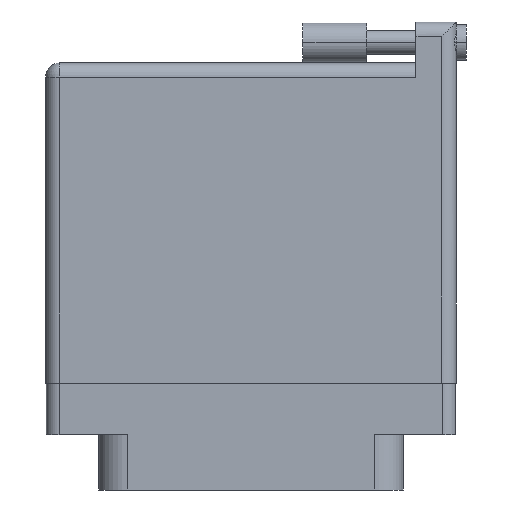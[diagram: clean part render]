
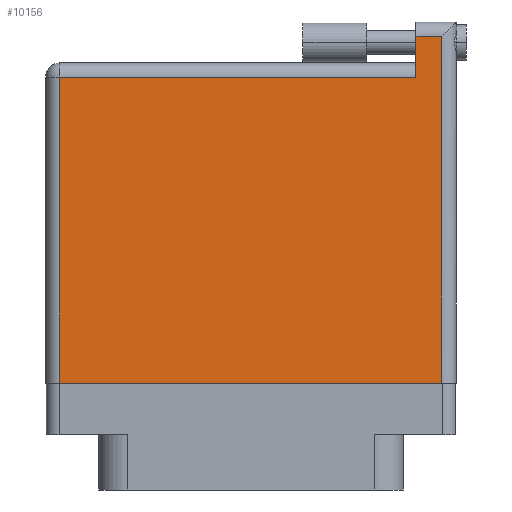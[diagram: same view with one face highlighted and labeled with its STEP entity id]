
A CAD part, front view. The second image highlights one B-rep face of the part: STEP entity #10156.
In plain terms, the highlighted face is planar.
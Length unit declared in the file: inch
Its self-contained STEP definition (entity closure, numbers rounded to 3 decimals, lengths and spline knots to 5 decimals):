
#523 = EDGE_CURVE ( 'NONE', #22296, #26404, #22113, .T. ) ;
#1125 = EDGE_CURVE ( 'NONE', #31940, #37923, #8595, .T. ) ;
#1723 = EDGE_CURVE ( 'NONE', #33157, #22296, #33054, .T. ) ;
#2141 = ORIENTED_EDGE ( 'NONE', *, *, #5294, .T. ) ;
#2783 = CARTESIAN_POINT ( 'NONE',  ( -0.934, -0.1, 0.4495 ) ) ;
#4022 = CARTESIAN_POINT ( 'NONE',  ( -0.934, -0.1, 0.4495 ) ) ;
#4082 = CARTESIAN_POINT ( 'NONE',  ( 0.934, 1.596, 0.4495 ) ) ;
#4830 = EDGE_CURVE ( 'NONE', #34901, #31940, #13661, .T. ) ;
#5192 = DIRECTION ( 'NONE',  ( 0., -1., 0. ) ) ;
#5294 = EDGE_CURVE ( 'NONE', #26404, #34901, #19897, .T. ) ;
#7741 = DIRECTION ( 'NONE',  ( -1., 0., 0. ) ) ;
#7782 = LINE ( 'NONE', #10392, #11637 ) ;
#8595 = LINE ( 'NONE', #8873, #16275 ) ;
#8873 = CARTESIAN_POINT ( 'NONE',  ( -1.004, -0.1, 0.4495 ) ) ;
#8925 = EDGE_CURVE ( 'NONE', #37923, #33157, #7782, .T. ) ;
#10156 = ADVANCED_FACE ( 'NONE', ( #24066 ), #29794, .F. ) ;
#10392 = CARTESIAN_POINT ( 'NONE',  ( 0.934, 1.666, 0.4495 ) ) ;
#11612 = CARTESIAN_POINT ( 'NONE',  ( 0.807, 1.596, 0.4495 ) ) ;
#11637 = VECTOR ( 'NONE', #13107, 39.37008 ) ;
#12786 = ORIENTED_EDGE ( 'NONE', *, *, #523, .T. ) ;
#12849 = VECTOR ( 'NONE', #7741, 39.37008 ) ;
#13107 = DIRECTION ( 'NONE',  ( 0., 1., 0. ) ) ;
#13513 = ORIENTED_EDGE ( 'NONE', *, *, #4830, .T. ) ;
#13623 = VECTOR ( 'NONE', #33402, 39.37008 ) ;
#13661 = LINE ( 'NONE', #2783, #19934 ) ;
#14086 = CARTESIAN_POINT ( 'NONE',  ( 0.807, 1.666, 0.4495 ) ) ;
#14533 = CARTESIAN_POINT ( 'NONE',  ( -1.004, 1.466, 0.4495 ) ) ;
#16275 = VECTOR ( 'NONE', #39687, 39.37008 ) ;
#17135 = CARTESIAN_POINT ( 'NONE',  ( -1.004, 1.596, 0.4495 ) ) ;
#17909 = CARTESIAN_POINT ( 'NONE',  ( 0.807, 1.396, 0.4495 ) ) ;
#17913 = DIRECTION ( 'NONE',  ( 0., 0., -1. ) ) ;
#18087 = CARTESIAN_POINT ( 'NONE',  ( -1.004, 1.396, 0.4495 ) ) ;
#19897 = LINE ( 'NONE', #18087, #13623 ) ;
#19934 = VECTOR ( 'NONE', #36561, 39.37008 ) ;
#20085 = ORIENTED_EDGE ( 'NONE', *, *, #8925, .T. ) ;
#20424 = AXIS2_PLACEMENT_3D ( 'NONE', #14533, #17913, #39315 ) ;
#22113 = LINE ( 'NONE', #14086, #22596 ) ;
#22274 = ORIENTED_EDGE ( 'NONE', *, *, #1723, .T. ) ;
#22296 = VERTEX_POINT ( 'NONE', #11612 ) ;
#22596 = VECTOR ( 'NONE', #5192, 39.37008 ) ;
#24066 = FACE_OUTER_BOUND ( 'NONE', #31773, .T. ) ;
#26404 = VERTEX_POINT ( 'NONE', #17909 ) ;
#29794 = PLANE ( 'NONE',  #20424 ) ;
#31312 = CARTESIAN_POINT ( 'NONE',  ( 0.934, -0.1, 0.4495 ) ) ;
#31773 = EDGE_LOOP ( 'NONE', ( #34555, #20085, #22274, #12786, #2141, #13513 ) ) ;
#31940 = VERTEX_POINT ( 'NONE', #4022 ) ;
#33054 = LINE ( 'NONE', #17135, #12849 ) ;
#33157 = VERTEX_POINT ( 'NONE', #4082 ) ;
#33402 = DIRECTION ( 'NONE',  ( -1., 0., 0. ) ) ;
#34555 = ORIENTED_EDGE ( 'NONE', *, *, #1125, .T. ) ;
#34901 = VERTEX_POINT ( 'NONE', #36477 ) ;
#36477 = CARTESIAN_POINT ( 'NONE',  ( -0.934, 1.396, 0.4495 ) ) ;
#36561 = DIRECTION ( 'NONE',  ( 0., -1., 0. ) ) ;
#37923 = VERTEX_POINT ( 'NONE', #31312 ) ;
#39315 = DIRECTION ( 'NONE',  ( -1., 0., 0. ) ) ;
#39687 = DIRECTION ( 'NONE',  ( 1., 0., 0. ) ) ;
